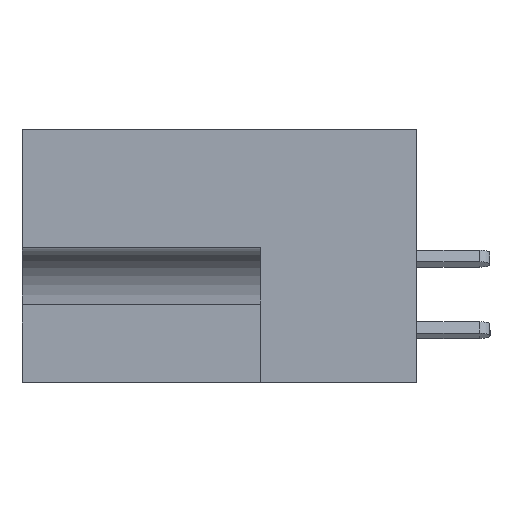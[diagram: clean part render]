
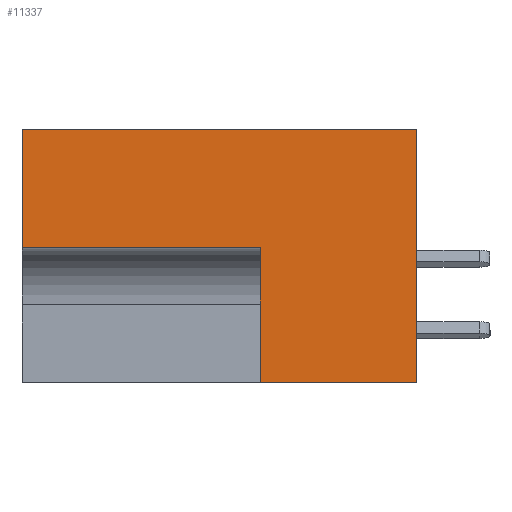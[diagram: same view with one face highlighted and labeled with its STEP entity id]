
A CAD part, left-side view. The second image highlights one B-rep face of the part: STEP entity #11337.
In plain terms, the highlighted planar face has unit normal (-1, 0, 0).
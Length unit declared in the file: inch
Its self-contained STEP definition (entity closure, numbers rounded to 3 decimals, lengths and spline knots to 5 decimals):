
#65 = ORIENTED_EDGE ( 'NONE', *, *, #25260, .F. ) ;
#1511 = EDGE_CURVE ( 'NONE', #7255, #12218, #3562, .T. ) ;
#1649 = CARTESIAN_POINT ( 'NONE',  ( 0., 0., -0.531 ) ) ;
#1712 = CARTESIAN_POINT ( 'NONE',  ( 0., 0., 0. ) ) ;
#3562 = LINE ( 'NONE', #5357, #27010 ) ;
#3907 = LINE ( 'NONE', #14259, #26967 ) ;
#5357 = CARTESIAN_POINT ( 'NONE',  ( 0., 0.453, -0.531 ) ) ;
#6107 = DIRECTION ( 'NONE',  ( 0., 0., 1. ) ) ;
#6735 = CARTESIAN_POINT ( 'NONE',  ( 0., 0.828, -0.248 ) ) ;
#7255 = VERTEX_POINT ( 'NONE', #10887 ) ;
#7573 = DIRECTION ( 'NONE',  ( 0., -1., 0. ) ) ;
#7961 = FACE_OUTER_BOUND ( 'NONE', #24550, .T. ) ;
#8161 = VERTEX_POINT ( 'NONE', #1712 ) ;
#10887 = CARTESIAN_POINT ( 'NONE',  ( 0., 0.328, -0.531 ) ) ;
#11078 = CARTESIAN_POINT ( 'NONE',  ( 0., 0.328, -0.248 ) ) ;
#11222 = CARTESIAN_POINT ( 'NONE',  ( 0., 0.828, 0. ) ) ;
#11337 = ADVANCED_FACE ( 'NONE', ( #7961 ), #16782, .F. ) ;
#12140 = AXIS2_PLACEMENT_3D ( 'NONE', #13872, #26431, #21632 ) ;
#12218 = VERTEX_POINT ( 'NONE', #1649 ) ;
#13047 = VERTEX_POINT ( 'NONE', #6735 ) ;
#13872 = CARTESIAN_POINT ( 'NONE',  ( 0., 0.453, 0. ) ) ;
#14259 = CARTESIAN_POINT ( 'NONE',  ( 0., 0.828, 0. ) ) ;
#14768 = CARTESIAN_POINT ( 'NONE',  ( 0., 0.328, -0.531 ) ) ;
#14907 = CARTESIAN_POINT ( 'NONE',  ( 0., 0.453, 0. ) ) ;
#15830 = LINE ( 'NONE', #18649, #26958 ) ;
#16197 = EDGE_CURVE ( 'NONE', #7255, #16419, #24746, .T. ) ;
#16419 = VERTEX_POINT ( 'NONE', #11078 ) ;
#16782 = PLANE ( 'NONE',  #12140 ) ;
#17447 = VECTOR ( 'NONE', #17467, 39.37008 ) ;
#17467 = DIRECTION ( 'NONE',  ( 0., 0., 1. ) ) ;
#17633 = DIRECTION ( 'NONE',  ( 0., -1., 0. ) ) ;
#17647 = EDGE_CURVE ( 'NONE', #16419, #13047, #15830, .T. ) ;
#18649 = CARTESIAN_POINT ( 'NONE',  ( 0., 0.328, -0.248 ) ) ;
#20428 = VECTOR ( 'NONE', #6107, 39.37008 ) ;
#20640 = CARTESIAN_POINT ( 'NONE',  ( 0., 0., 0. ) ) ;
#21027 = DIRECTION ( 'NONE',  ( 0., 1., 0. ) ) ;
#21632 = DIRECTION ( 'NONE',  ( 0., 0., -1. ) ) ;
#22877 = LINE ( 'NONE', #14907, #28608 ) ;
#24172 = DIRECTION ( 'NONE',  ( 0., 0., 1. ) ) ;
#24550 = EDGE_LOOP ( 'NONE', ( #65, #28782, #28903, #27510, #26106, #24710 ) ) ;
#24710 = ORIENTED_EDGE ( 'NONE', *, *, #28827, .F. ) ;
#24746 = LINE ( 'NONE', #14768, #17447 ) ;
#25260 = EDGE_CURVE ( 'NONE', #13047, #28025, #3907, .T. ) ;
#25901 = EDGE_CURVE ( 'NONE', #12218, #8161, #28842, .T. ) ;
#26106 = ORIENTED_EDGE ( 'NONE', *, *, #25901, .T. ) ;
#26431 = DIRECTION ( 'NONE',  ( 1., 0., 0. ) ) ;
#26958 = VECTOR ( 'NONE', #21027, 39.37008 ) ;
#26967 = VECTOR ( 'NONE', #24172, 39.37008 ) ;
#27010 = VECTOR ( 'NONE', #17633, 39.37008 ) ;
#27510 = ORIENTED_EDGE ( 'NONE', *, *, #1511, .T. ) ;
#28025 = VERTEX_POINT ( 'NONE', #11222 ) ;
#28608 = VECTOR ( 'NONE', #7573, 39.37008 ) ;
#28782 = ORIENTED_EDGE ( 'NONE', *, *, #17647, .F. ) ;
#28827 = EDGE_CURVE ( 'NONE', #28025, #8161, #22877, .T. ) ;
#28842 = LINE ( 'NONE', #20640, #20428 ) ;
#28903 = ORIENTED_EDGE ( 'NONE', *, *, #16197, .F. ) ;
